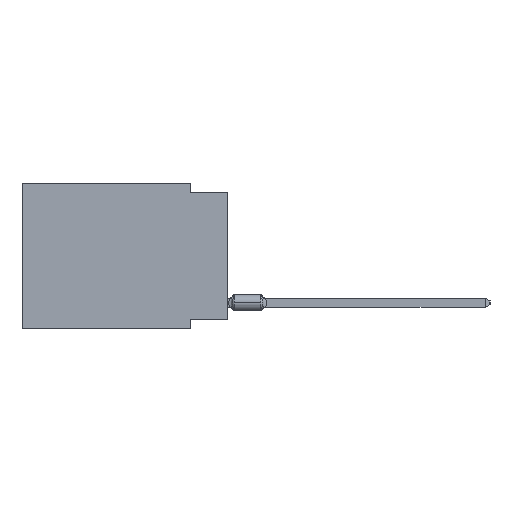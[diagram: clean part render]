
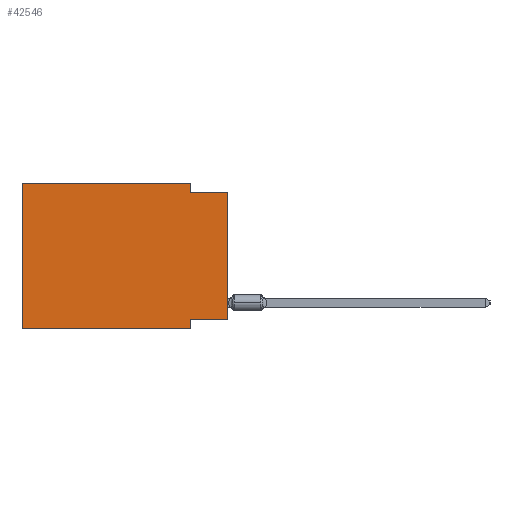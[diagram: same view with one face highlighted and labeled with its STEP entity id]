
A CAD part, left-side view. The second image highlights one B-rep face of the part: STEP entity #42546.
In plain terms, the highlighted planar face has unit normal (-1, 0, 0).
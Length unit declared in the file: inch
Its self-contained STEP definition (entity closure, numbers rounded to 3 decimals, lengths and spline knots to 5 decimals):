
#789 = LINE ( 'NONE', #20557, #46064 ) ;
#1841 = VERTEX_POINT ( 'NONE', #14509 ) ;
#2253 = EDGE_CURVE ( 'NONE', #52276, #74726, #789, .T. ) ;
#4742 = DIRECTION ( 'NONE',  ( 0., 0., 1. ) ) ;
#5444 = EDGE_LOOP ( 'NONE', ( #14504, #43503, #70627, #15173, #43782, #34180, #33326, #16656 ) ) ;
#5886 = DIRECTION ( 'NONE',  ( 0., 0., 1. ) ) ;
#5914 = CARTESIAN_POINT ( 'NONE',  ( 0., 0.1, -0.39 ) ) ;
#7870 = CARTESIAN_POINT ( 'NONE',  ( 0., 0.55, 0. ) ) ;
#9187 = CARTESIAN_POINT ( 'NONE',  ( 0., 0.1, -0.39 ) ) ;
#9783 = DIRECTION ( 'NONE',  ( 0., 0., -1. ) ) ;
#11224 = LINE ( 'NONE', #5914, #38358 ) ;
#13506 = VERTEX_POINT ( 'NONE', #55574 ) ;
#14002 = EDGE_CURVE ( 'NONE', #1841, #52276, #38215, .T. ) ;
#14504 = ORIENTED_EDGE ( 'NONE', *, *, #67362, .T. ) ;
#14509 = CARTESIAN_POINT ( 'NONE',  ( 0., 0.55, 0. ) ) ;
#14536 = CARTESIAN_POINT ( 'NONE',  ( 0., 0.55, -0.39 ) ) ;
#15173 = ORIENTED_EDGE ( 'NONE', *, *, #14002, .F. ) ;
#15761 = LINE ( 'NONE', #56097, #38547 ) ;
#16371 = FACE_OUTER_BOUND ( 'NONE', #5444, .T. ) ;
#16640 = DIRECTION ( 'NONE',  ( 0., 1., 0. ) ) ;
#16656 = ORIENTED_EDGE ( 'NONE', *, *, #81223, .F. ) ;
#17466 = VERTEX_POINT ( 'NONE', #9187 ) ;
#18376 = CARTESIAN_POINT ( 'NONE',  ( 0., 0., -0.365 ) ) ;
#20126 = DIRECTION ( 'NONE',  ( 0., 0., -1. ) ) ;
#20382 = CARTESIAN_POINT ( 'NONE',  ( 0., 0.1, 0. ) ) ;
#20557 = CARTESIAN_POINT ( 'NONE',  ( 0., 0.1, 0. ) ) ;
#20800 = DIRECTION ( 'NONE',  ( 0., -1., 0. ) ) ;
#21644 = LINE ( 'NONE', #27803, #65249 ) ;
#25918 = CARTESIAN_POINT ( 'NONE',  ( 0., 0.55, 0. ) ) ;
#25955 = EDGE_CURVE ( 'NONE', #33844, #17466, #11224, .T. ) ;
#27803 = CARTESIAN_POINT ( 'NONE',  ( 0., 0., -0.025 ) ) ;
#31336 = LINE ( 'NONE', #65554, #64891 ) ;
#31569 = EDGE_CURVE ( 'NONE', #45186, #17466, #15761, .T. ) ;
#33326 = ORIENTED_EDGE ( 'NONE', *, *, #25955, .F. ) ;
#33844 = VERTEX_POINT ( 'NONE', #54236 ) ;
#34180 = ORIENTED_EDGE ( 'NONE', *, *, #31569, .T. ) ;
#35746 = CARTESIAN_POINT ( 'NONE',  ( 0., 0.1, -0.025 ) ) ;
#37440 = VECTOR ( 'NONE', #66732, 39.37008 ) ;
#38215 = LINE ( 'NONE', #25918, #37440 ) ;
#38358 = VECTOR ( 'NONE', #45400, 39.37008 ) ;
#38547 = VECTOR ( 'NONE', #81981, 39.37008 ) ;
#42546 = ADVANCED_FACE ( 'NONE', ( #16371 ), #43970, .F. ) ;
#43100 = CARTESIAN_POINT ( 'NONE',  ( 0., 0.55, 0. ) ) ;
#43503 = ORIENTED_EDGE ( 'NONE', *, *, #84666, .F. ) ;
#43782 = ORIENTED_EDGE ( 'NONE', *, *, #79936, .F. ) ;
#43970 = PLANE ( 'NONE',  #86177 ) ;
#45186 = VERTEX_POINT ( 'NONE', #14536 ) ;
#45400 = DIRECTION ( 'NONE',  ( 0., 0., -1. ) ) ;
#46064 = VECTOR ( 'NONE', #20126, 39.37008 ) ;
#51704 = VERTEX_POINT ( 'NONE', #64064 ) ;
#52276 = VERTEX_POINT ( 'NONE', #20382 ) ;
#54236 = CARTESIAN_POINT ( 'NONE',  ( 0., 0.1, -0.365 ) ) ;
#55574 = CARTESIAN_POINT ( 'NONE',  ( 0., 0., -0.025 ) ) ;
#56097 = CARTESIAN_POINT ( 'NONE',  ( 0., 0.55, -0.39 ) ) ;
#57397 = LINE ( 'NONE', #18376, #68552 ) ;
#64064 = CARTESIAN_POINT ( 'NONE',  ( 0., 0., -0.365 ) ) ;
#64891 = VECTOR ( 'NONE', #5886, 39.37008 ) ;
#65249 = VECTOR ( 'NONE', #20800, 39.37008 ) ;
#65554 = CARTESIAN_POINT ( 'NONE',  ( 0., 0., 0. ) ) ;
#66732 = DIRECTION ( 'NONE',  ( 0., -1., 0. ) ) ;
#67362 = EDGE_CURVE ( 'NONE', #51704, #13506, #31336, .T. ) ;
#67978 = LINE ( 'NONE', #7870, #86593 ) ;
#68552 = VECTOR ( 'NONE', #16640, 39.37008 ) ;
#70296 = DIRECTION ( 'NONE',  ( 1., 0., 0. ) ) ;
#70627 = ORIENTED_EDGE ( 'NONE', *, *, #2253, .F. ) ;
#74726 = VERTEX_POINT ( 'NONE', #35746 ) ;
#79936 = EDGE_CURVE ( 'NONE', #45186, #1841, #67978, .T. ) ;
#81223 = EDGE_CURVE ( 'NONE', #51704, #33844, #57397, .T. ) ;
#81981 = DIRECTION ( 'NONE',  ( 0., -1., 0. ) ) ;
#84666 = EDGE_CURVE ( 'NONE', #74726, #13506, #21644, .T. ) ;
#86177 = AXIS2_PLACEMENT_3D ( 'NONE', #43100, #70296, #9783 ) ;
#86593 = VECTOR ( 'NONE', #4742, 39.37008 ) ;
